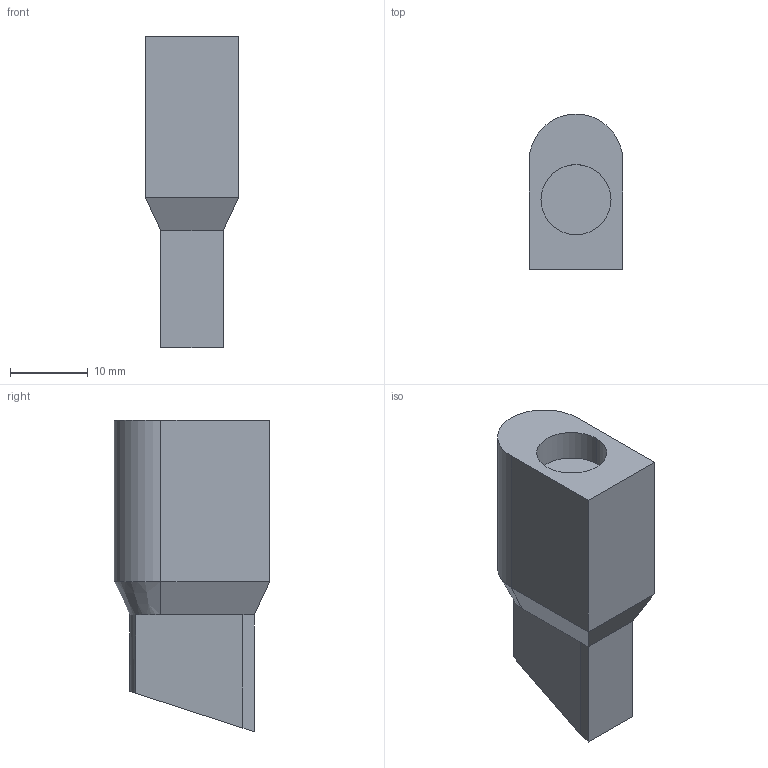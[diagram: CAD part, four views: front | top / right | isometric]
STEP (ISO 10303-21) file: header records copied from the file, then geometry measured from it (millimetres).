
FILE_DESCRIPTION (( 'STEP AP214' ), '1' );
FILE_NAME ('Plunger 2.0 5.56.STEP', '2025-05-18T10:37:43', ( '' ), ( '' ), 'SwSTEP 2.0', 'SolidWorks 2024', '' );
FILE_SCHEMA (( 'AUTOMOTIVE_DESIGN' ));
Length unit declared in the file: millimetre
Products named in the file (1): Plunger 2.0 5.56
Bounding box: 12 x 20 x 40 mm (x, y, z)
Volume: 6418.4 mm3; surface area: 2481.4 mm2
Topology: 1 solids, 1 shells, 21 faces, 44 edges, 26 vertices
Faces by surface type: plane 16, cylinder 4, cone 1
Entity records: 570 total; most frequent: DIRECTION 96, CARTESIAN_POINT 95, ORIENTED_EDGE 88, EDGE_CURVE 44, LINE 34, VECTOR 34, AXIS2_PLACEMENT_3D 31, VERTEX_POINT 26
